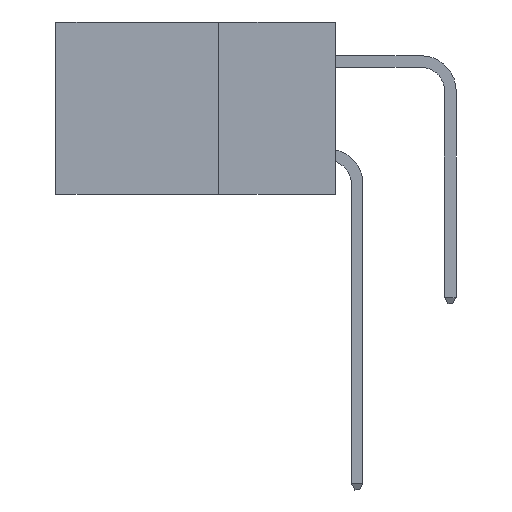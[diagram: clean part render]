
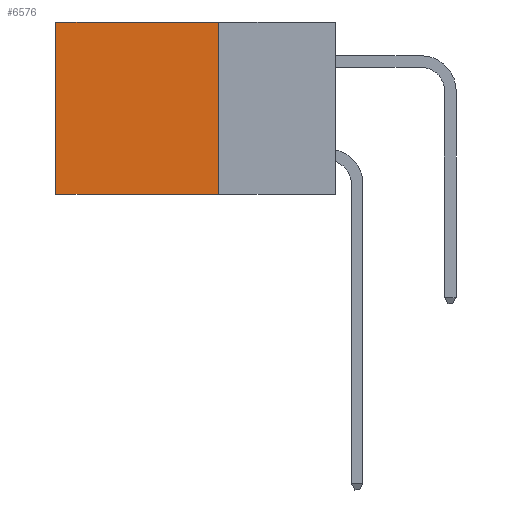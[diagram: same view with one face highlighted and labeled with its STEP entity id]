
A CAD part, left-side view. The second image highlights one B-rep face of the part: STEP entity #6576.
In plain terms, the highlighted planar face has unit normal (-1, 0, 0).
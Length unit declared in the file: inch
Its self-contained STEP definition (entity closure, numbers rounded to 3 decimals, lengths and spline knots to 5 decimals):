
#17 = ORIENTED_EDGE ( 'NONE', *, *, #1487, .F. ) ;
#97 = VECTOR ( 'NONE', #8437, 39.37008 ) ;
#214 = DIRECTION ( 'NONE',  ( 0., 0., -1. ) ) ;
#371 = VERTEX_POINT ( 'NONE', #1840 ) ;
#1072 = ORIENTED_EDGE ( 'NONE', *, *, #3251, .T. ) ;
#1436 = CARTESIAN_POINT ( 'NONE',  ( 0.2875, 0.25, 0. ) ) ;
#1487 = EDGE_CURVE ( 'NONE', #13934, #371, #8493, .T. ) ;
#1639 = VECTOR ( 'NONE', #11094, 39.37008 ) ;
#1840 = CARTESIAN_POINT ( 'NONE',  ( 0.2875, 0.6, -0.37 ) ) ;
#2726 = VERTEX_POINT ( 'NONE', #11827 ) ;
#2864 = VECTOR ( 'NONE', #11718, 39.37008 ) ;
#2975 = VERTEX_POINT ( 'NONE', #12229 ) ;
#3251 = EDGE_CURVE ( 'NONE', #2975, #2726, #11398, .T. ) ;
#3300 = CARTESIAN_POINT ( 'NONE',  ( 0.2875, 0.25, 0. ) ) ;
#3733 = PLANE ( 'NONE',  #12105 ) ;
#6576 = ADVANCED_FACE ( 'NONE', ( #13016 ), #3733, .F. ) ;
#7137 = DIRECTION ( 'NONE',  ( 1., 0., 0. ) ) ;
#8437 = DIRECTION ( 'NONE',  ( 0., 0., -1. ) ) ;
#8486 = CARTESIAN_POINT ( 'NONE',  ( 0.2875, 0.6, 0. ) ) ;
#8493 = LINE ( 'NONE', #11734, #2864 ) ;
#8502 = VECTOR ( 'NONE', #14031, 39.37008 ) ;
#9479 = ORIENTED_EDGE ( 'NONE', *, *, #9763, .T. ) ;
#9763 = EDGE_CURVE ( 'NONE', #2726, #371, #12141, .T. ) ;
#10273 = LINE ( 'NONE', #3300, #1639 ) ;
#10462 = EDGE_CURVE ( 'NONE', #2975, #13934, #10273, .T. ) ;
#10679 = ORIENTED_EDGE ( 'NONE', *, *, #10462, .F. ) ;
#11094 = DIRECTION ( 'NONE',  ( 0., 0., -1. ) ) ;
#11398 = LINE ( 'NONE', #14401, #8502 ) ;
#11718 = DIRECTION ( 'NONE',  ( 0., 1., 0. ) ) ;
#11734 = CARTESIAN_POINT ( 'NONE',  ( 0.2875, 0.25, -0.37 ) ) ;
#11800 = CARTESIAN_POINT ( 'NONE',  ( 0.2875, 0.25, -0.37 ) ) ;
#11827 = CARTESIAN_POINT ( 'NONE',  ( 0.2875, 0.6, 0. ) ) ;
#11948 = EDGE_LOOP ( 'NONE', ( #9479, #17, #10679, #1072 ) ) ;
#12105 = AXIS2_PLACEMENT_3D ( 'NONE', #1436, #7137, #214 ) ;
#12141 = LINE ( 'NONE', #8486, #97 ) ;
#12229 = CARTESIAN_POINT ( 'NONE',  ( 0.2875, 0.25, 0. ) ) ;
#13016 = FACE_OUTER_BOUND ( 'NONE', #11948, .T. ) ;
#13934 = VERTEX_POINT ( 'NONE', #11800 ) ;
#14031 = DIRECTION ( 'NONE',  ( 0., 1., 0. ) ) ;
#14401 = CARTESIAN_POINT ( 'NONE',  ( 0.2875, 0.25, 0. ) ) ;
